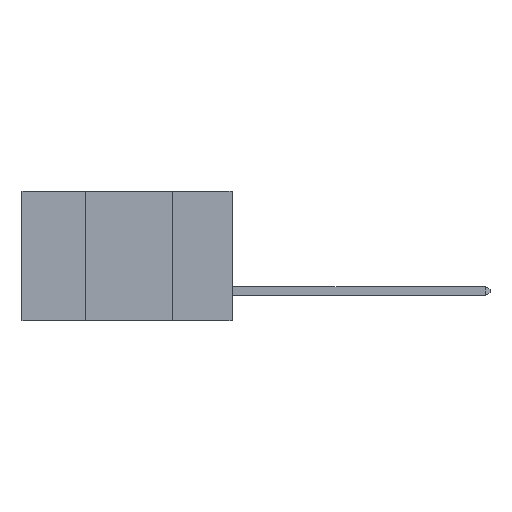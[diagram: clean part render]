
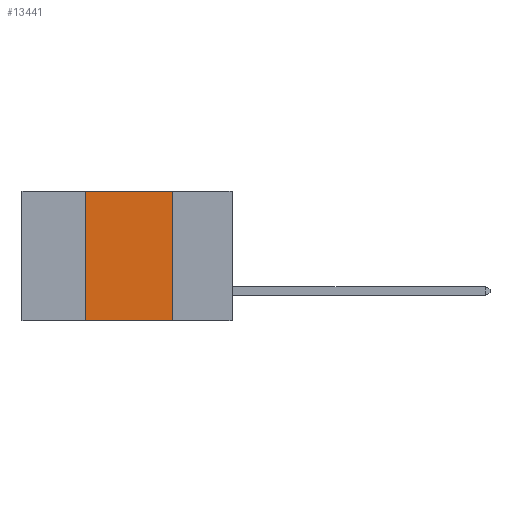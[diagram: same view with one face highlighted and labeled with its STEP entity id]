
A CAD part, left-side view. The second image highlights one B-rep face of the part: STEP entity #13441.
In plain terms, the highlighted planar face has unit normal (-1, 0, 0).
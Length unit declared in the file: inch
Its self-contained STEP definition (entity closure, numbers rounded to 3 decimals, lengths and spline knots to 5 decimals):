
#3 = CARTESIAN_POINT ( 'NONE',  ( 0., 0.17, -0.37 ) ) ;
#421 = ORIENTED_EDGE ( 'NONE', *, *, #14216, .F. ) ;
#659 = DIRECTION ( 'NONE',  ( 0., 0., 1. ) ) ;
#719 = EDGE_CURVE ( 'NONE', #9374, #8067, #13269, .T. ) ;
#2345 = LINE ( 'NONE', #8316, #10723 ) ;
#2355 = LINE ( 'NONE', #3676, #7804 ) ;
#3085 = PLANE ( 'NONE',  #11333 ) ;
#3514 = VERTEX_POINT ( 'NONE', #13013 ) ;
#3584 = DIRECTION ( 'NONE',  ( 0., -1., 0. ) ) ;
#3664 = CARTESIAN_POINT ( 'NONE',  ( 0., 0.17, 0. ) ) ;
#3676 = CARTESIAN_POINT ( 'NONE',  ( 0., 0.6, -0.37 ) ) ;
#3721 = CARTESIAN_POINT ( 'NONE',  ( 0., 0.17, 0. ) ) ;
#4498 = FACE_OUTER_BOUND ( 'NONE', #12503, .T. ) ;
#4692 = EDGE_CURVE ( 'NONE', #14093, #8067, #2355, .T. ) ;
#5011 = DIRECTION ( 'NONE',  ( 0., -1., 0. ) ) ;
#5262 = DIRECTION ( 'NONE',  ( 0., 0., -1. ) ) ;
#5704 = VECTOR ( 'NONE', #5011, 39.37008 ) ;
#6052 = LINE ( 'NONE', #13837, #5704 ) ;
#7488 = ORIENTED_EDGE ( 'NONE', *, *, #4692, .T. ) ;
#7804 = VECTOR ( 'NONE', #3584, 39.37008 ) ;
#8067 = VERTEX_POINT ( 'NONE', #3 ) ;
#8316 = CARTESIAN_POINT ( 'NONE',  ( 0., 0.42, 0. ) ) ;
#8359 = DIRECTION ( 'NONE',  ( 0., 0., -1. ) ) ;
#9200 = CARTESIAN_POINT ( 'NONE',  ( 0., 0.42, -0.37 ) ) ;
#9374 = VERTEX_POINT ( 'NONE', #3721 ) ;
#9530 = EDGE_CURVE ( 'NONE', #14093, #3514, #2345, .T. ) ;
#9952 = VECTOR ( 'NONE', #8359, 39.37008 ) ;
#10292 = ORIENTED_EDGE ( 'NONE', *, *, #719, .F. ) ;
#10699 = ORIENTED_EDGE ( 'NONE', *, *, #9530, .F. ) ;
#10723 = VECTOR ( 'NONE', #659, 39.37008 ) ;
#10730 = CARTESIAN_POINT ( 'NONE',  ( 0., 0.6, 0. ) ) ;
#11333 = AXIS2_PLACEMENT_3D ( 'NONE', #10730, #11852, #5262 ) ;
#11852 = DIRECTION ( 'NONE',  ( 1., 0., 0. ) ) ;
#12503 = EDGE_LOOP ( 'NONE', ( #10292, #421, #10699, #7488 ) ) ;
#13013 = CARTESIAN_POINT ( 'NONE',  ( 0., 0.42, 0. ) ) ;
#13269 = LINE ( 'NONE', #3664, #9952 ) ;
#13441 = ADVANCED_FACE ( 'NONE', ( #4498 ), #3085, .F. ) ;
#13837 = CARTESIAN_POINT ( 'NONE',  ( 0., 0.6, 0. ) ) ;
#14093 = VERTEX_POINT ( 'NONE', #9200 ) ;
#14216 = EDGE_CURVE ( 'NONE', #3514, #9374, #6052, .T. ) ;
